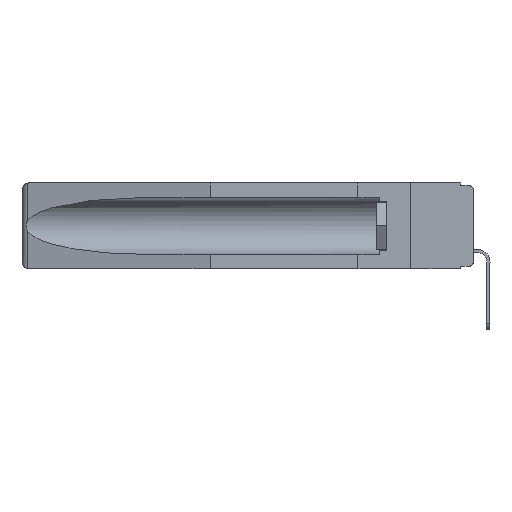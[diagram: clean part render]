
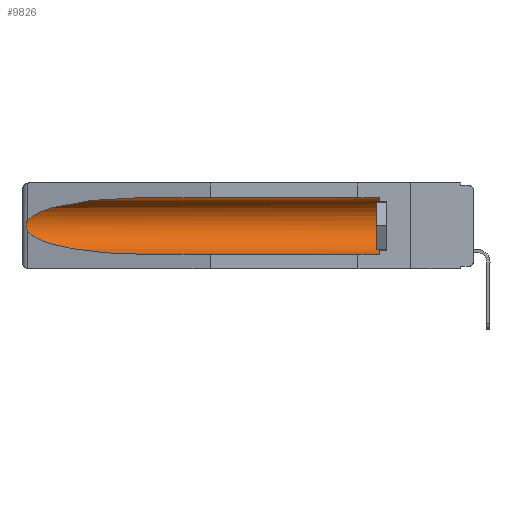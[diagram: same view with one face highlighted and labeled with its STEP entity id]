
A CAD part, left-side view. The second image highlights one B-rep face of the part: STEP entity #9826.
In plain terms, the highlighted cylindrical face has radius 2.857 mm (diameter 5.715 mm), a partial arc.
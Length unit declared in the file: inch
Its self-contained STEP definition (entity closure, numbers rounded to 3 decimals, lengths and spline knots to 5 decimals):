
#898 = EDGE_CURVE ( 'NONE', #16941, #14572, #17884, .T. ) ;
#1068 = VECTOR ( 'NONE', #13842, 39.37008 ) ;
#1577 = DIRECTION ( 'NONE',  ( 0., 1., 0. ) ) ;
#1644 = EDGE_CURVE ( 'NONE', #14272, #12873, #17709, .T. ) ;
#1695 = CARTESIAN_POINT ( 'NONE',  ( 0.26654, 1.53092, -0.15636 ) ) ;
#1876 = CARTESIAN_POINT ( 'NONE',  ( 0.155, 1.07973, -0.059 ) ) ;
#1894 = CARTESIAN_POINT ( 'NONE',  ( 0.2673, 1.53269, -0.17917 ) ) ;
#2277 = EDGE_CURVE ( 'NONE', #16995, #18347, #7547, .T. ) ;
#3204 = CARTESIAN_POINT ( 'NONE',  ( 0.155, -0.30754, -0.1715 ) ) ;
#3246 = CARTESIAN_POINT ( 'NONE',  ( 0.21114, 1.30732, -0.284 ) ) ;
#3374 = CARTESIAN_POINT ( 'NONE',  ( 0.2675, 1.53308, -0.16763 ) ) ;
#3468 = CARTESIAN_POINT ( 'NONE',  ( 0.26655, 1.53094, -0.18657 ) ) ;
#6080 = EDGE_LOOP ( 'NONE', ( #12931, #16655, #9031, #13922, #8449, #18940 ) ) ;
#6234 = CARTESIAN_POINT ( 'NONE',  ( 0.26537, 1.52718, -0.19328 ) ) ;
#6331 = CARTESIAN_POINT ( 'NONE',  ( 0.155, 0.126, -0.1715 ) ) ;
#6398 = B_SPLINE_CURVE_WITH_KNOTS ( 'NONE', 3,
 ( #6546, #16886, #1695, #11002, #3374, #15201, #1894, #3468, #15594, #9323 ),
 .UNSPECIFIED., .F., .F.,
 ( 4, 2, 2, 2, 4 ),
 ( 0., 0.00029, 0.00058, 0.00087, 0.00117 ),
 .UNSPECIFIED. ) ;
#6546 = CARTESIAN_POINT ( 'NONE',  ( 0.26537, 1.52718, -0.14972 ) ) ;
#6646 = AXIS2_PLACEMENT_3D ( 'NONE', #3204, #7862, #18387 ) ;
#7547 =( BOUNDED_CURVE ( )  B_SPLINE_CURVE ( 3, ( #6234, #12158, #3246, #7905 ),
 .UNSPECIFIED., .F., .T. ) 
 B_SPLINE_CURVE_WITH_KNOTS ( ( 4, 4 ),
 ( 0.1948, 1.5708 ),
 .UNSPECIFIED. ) 
 CURVE ( )  GEOMETRIC_REPRESENTATION_ITEM ( )  RATIONAL_B_SPLINE_CURVE ( ( 1., 0.848, 0.848, 1. ) ) 
 REPRESENTATION_ITEM ( '' )  );
#7767 = FACE_OUTER_BOUND ( 'NONE', #6080, .T. ) ;
#7862 = DIRECTION ( 'NONE',  ( 0., 1., 0. ) ) ;
#7905 = CARTESIAN_POINT ( 'NONE',  ( 0.155, 1.07973, -0.284 ) ) ;
#8449 = ORIENTED_EDGE ( 'NONE', *, *, #898, .T. ) ;
#8733 = CARTESIAN_POINT ( 'NONE',  ( 0.155, 1.07973, -0.059 ) ) ;
#9031 = ORIENTED_EDGE ( 'NONE', *, *, #2277, .T. ) ;
#9274 = CARTESIAN_POINT ( 'NONE',  ( 0.155, 0.126, -0.059 ) ) ;
#9290 = LINE ( 'NONE', #13821, #14326 ) ;
#9323 = CARTESIAN_POINT ( 'NONE',  ( 0.26537, 1.52718, -0.19328 ) ) ;
#9826 = ADVANCED_FACE ( 'NONE', ( #7767 ), #13793, .F. ) ;
#10228 = CARTESIAN_POINT ( 'NONE',  ( 0.25451, 1.48313, -0.09465 ) ) ;
#11002 = CARTESIAN_POINT ( 'NONE',  ( 0.2673, 1.5327, -0.16383 ) ) ;
#11298 = CARTESIAN_POINT ( 'NONE',  ( 0.155, 0.126, -0.284 ) ) ;
#11745 = EDGE_CURVE ( 'NONE', #16941, #18347, #15023, .T. ) ;
#12158 = CARTESIAN_POINT ( 'NONE',  ( 0.25451, 1.48313, -0.24835 ) ) ;
#12346 = DIRECTION ( 'NONE',  ( 0., -1., 0. ) ) ;
#12873 = VERTEX_POINT ( 'NONE', #18650 ) ;
#12931 = ORIENTED_EDGE ( 'NONE', *, *, #1644, .T. ) ;
#13034 = CARTESIAN_POINT ( 'NONE',  ( 0.26537, 1.52718, -0.19328 ) ) ;
#13544 = CARTESIAN_POINT ( 'NONE',  ( 0.155, 1.07973, -0.284 ) ) ;
#13639 = CARTESIAN_POINT ( 'NONE',  ( 0.155, -0.30754, -0.284 ) ) ;
#13793 = CYLINDRICAL_SURFACE ( 'NONE', #6646, 0.1125 ) ;
#13821 = CARTESIAN_POINT ( 'NONE',  ( 0.155, -0.30754, -0.059 ) ) ;
#13842 = DIRECTION ( 'NONE',  ( 0., 1., 0. ) ) ;
#13922 = ORIENTED_EDGE ( 'NONE', *, *, #11745, .F. ) ;
#14272 = VERTEX_POINT ( 'NONE', #1876 ) ;
#14326 = VECTOR ( 'NONE', #1577, 39.37008 ) ;
#14572 = VERTEX_POINT ( 'NONE', #9274 ) ;
#15023 = LINE ( 'NONE', #13639, #1068 ) ;
#15201 = CARTESIAN_POINT ( 'NONE',  ( 0.2675, 1.53308, -0.17534 ) ) ;
#15551 = EDGE_CURVE ( 'NONE', #12873, #16995, #6398, .T. ) ;
#15594 = CARTESIAN_POINT ( 'NONE',  ( 0.26597, 1.5296, -0.19026 ) ) ;
#16655 = ORIENTED_EDGE ( 'NONE', *, *, #15551, .T. ) ;
#16868 = DIRECTION ( 'NONE',  ( 0., 0., 1. ) ) ;
#16886 = CARTESIAN_POINT ( 'NONE',  ( 0.26597, 1.52961, -0.15275 ) ) ;
#16941 = VERTEX_POINT ( 'NONE', #11298 ) ;
#16995 = VERTEX_POINT ( 'NONE', #13034 ) ;
#17550 = EDGE_CURVE ( 'NONE', #14572, #14272, #9290, .T. ) ;
#17667 = CARTESIAN_POINT ( 'NONE',  ( 0.21114, 1.30732, -0.059 ) ) ;
#17709 =( BOUNDED_CURVE ( )  B_SPLINE_CURVE ( 3, ( #8733, #17667, #10228, #19243 ),
 .UNSPECIFIED., .F., .T. ) 
 B_SPLINE_CURVE_WITH_KNOTS ( ( 4, 4 ),
 ( 4.71239, 6.08839 ),
 .UNSPECIFIED. ) 
 CURVE ( )  GEOMETRIC_REPRESENTATION_ITEM ( )  RATIONAL_B_SPLINE_CURVE ( ( 1., 0.848, 0.848, 1. ) ) 
 REPRESENTATION_ITEM ( '' )  );
#17884 = CIRCLE ( 'NONE', #19454, 0.1125 ) ;
#18347 = VERTEX_POINT ( 'NONE', #13544 ) ;
#18387 = DIRECTION ( 'NONE',  ( 0., 0., 1. ) ) ;
#18650 = CARTESIAN_POINT ( 'NONE',  ( 0.26537, 1.52718, -0.14972 ) ) ;
#18940 = ORIENTED_EDGE ( 'NONE', *, *, #17550, .T. ) ;
#19243 = CARTESIAN_POINT ( 'NONE',  ( 0.26537, 1.52718, -0.14972 ) ) ;
#19454 = AXIS2_PLACEMENT_3D ( 'NONE', #6331, #12346, #16868 ) ;
